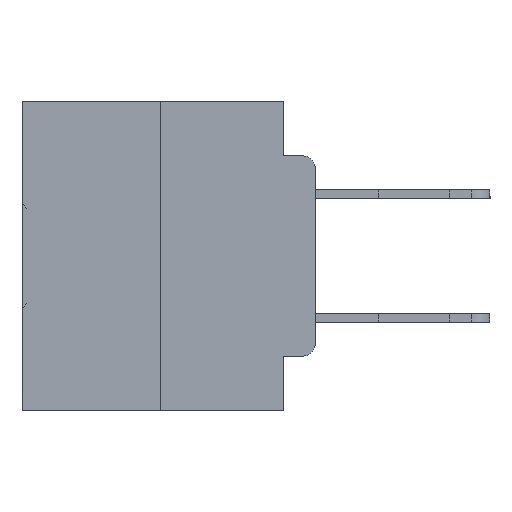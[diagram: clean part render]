
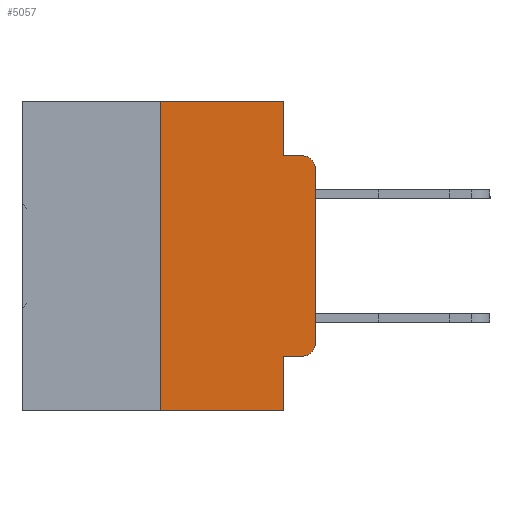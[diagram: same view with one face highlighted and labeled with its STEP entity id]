
A CAD part, left-side view. The second image highlights one B-rep face of the part: STEP entity #5057.
In plain terms, the highlighted planar face has unit normal (-1, 0, 0).
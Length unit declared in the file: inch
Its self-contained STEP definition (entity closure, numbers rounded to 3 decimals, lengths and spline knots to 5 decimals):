
#38 = VERTEX_POINT ( 'NONE', #27426 ) ;
#73 = EDGE_CURVE ( 'NONE', #22135, #20556, #468, .T. ) ;
#468 = CIRCLE ( 'NONE', #27942, 0.02 ) ;
#1991 = VERTEX_POINT ( 'NONE', #22120 ) ;
#2559 = DIRECTION ( 'NONE',  ( 0., 0., -1. ) ) ;
#2603 = CARTESIAN_POINT ( 'NONE',  ( 0., 0.02, -0.0885 ) ) ;
#2641 = VERTEX_POINT ( 'NONE', #11782 ) ;
#2790 = VECTOR ( 'NONE', #2559, 39.37008 ) ;
#3062 = ORIENTED_EDGE ( 'NONE', *, *, #28725, .F. ) ;
#3440 = CARTESIAN_POINT ( 'NONE',  ( 0., 0.25, 0. ) ) ;
#4510 = EDGE_CURVE ( 'NONE', #1991, #26244, #28996, .T. ) ;
#5057 = ADVANCED_FACE ( 'NONE', ( #19769 ), #16240, .F. ) ;
#5175 = ORIENTED_EDGE ( 'NONE', *, *, #10488, .F. ) ;
#5208 = CARTESIAN_POINT ( 'NONE',  ( 0., 0.02, -0.3915 ) ) ;
#5352 = CARTESIAN_POINT ( 'NONE',  ( 0., 0.051, 0. ) ) ;
#5661 = LINE ( 'NONE', #27698, #26513 ) ;
#6162 = ORIENTED_EDGE ( 'NONE', *, *, #22322, .T. ) ;
#6453 = EDGE_LOOP ( 'NONE', ( #10650, #28845, #28217, #3062, #5175, #31381, #14364, #29617, #17649, #6162 ) ) ;
#6769 = CARTESIAN_POINT ( 'NONE',  ( 0., 0.051, -0.4115 ) ) ;
#6932 = CIRCLE ( 'NONE', #30963, 0.02 ) ;
#7914 = DIRECTION ( 'NONE',  ( 0., 0., -1. ) ) ;
#8306 = VECTOR ( 'NONE', #17168, 39.37008 ) ;
#8898 = AXIS2_PLACEMENT_3D ( 'NONE', #13912, #11565, #14212 ) ;
#9503 = DIRECTION ( 'NONE',  ( 0., -1., 0. ) ) ;
#9935 = LINE ( 'NONE', #33737, #2790 ) ;
#10488 = EDGE_CURVE ( 'NONE', #26244, #26104, #29920, .T. ) ;
#10646 = DIRECTION ( 'NONE',  ( 0., -1., 0. ) ) ;
#10650 = ORIENTED_EDGE ( 'NONE', *, *, #28470, .T. ) ;
#11565 = DIRECTION ( 'NONE',  ( 1., 0., 0. ) ) ;
#11782 = CARTESIAN_POINT ( 'NONE',  ( 0., 0.02, -0.4115 ) ) ;
#12113 = VERTEX_POINT ( 'NONE', #20644 ) ;
#12252 = DIRECTION ( 'NONE',  ( 0., -1., 0. ) ) ;
#12771 = EDGE_CURVE ( 'NONE', #26099, #12113, #9935, .T. ) ;
#13738 = EDGE_CURVE ( 'NONE', #1991, #12113, #5661, .T. ) ;
#13912 = CARTESIAN_POINT ( 'NONE',  ( 0., 0.473, 0. ) ) ;
#14031 = CARTESIAN_POINT ( 'NONE',  ( 0., 0., -0.3915 ) ) ;
#14212 = DIRECTION ( 'NONE',  ( 0., 0., -1. ) ) ;
#14364 = ORIENTED_EDGE ( 'NONE', *, *, #13738, .T. ) ;
#14408 = DIRECTION ( 'NONE',  ( 0., -1., 0. ) ) ;
#14511 = LINE ( 'NONE', #6769, #20534 ) ;
#16130 = CARTESIAN_POINT ( 'NONE',  ( 0., 0.051, -0.4115 ) ) ;
#16240 = PLANE ( 'NONE',  #8898 ) ;
#17139 = CARTESIAN_POINT ( 'NONE',  ( 0., 0.25, 0. ) ) ;
#17168 = DIRECTION ( 'NONE',  ( 0., 0., 1. ) ) ;
#17247 = EDGE_CURVE ( 'NONE', #26099, #2641, #14511, .T. ) ;
#17649 = ORIENTED_EDGE ( 'NONE', *, *, #17247, .T. ) ;
#18200 = CARTESIAN_POINT ( 'NONE',  ( 0., 0., 0. ) ) ;
#19360 = VECTOR ( 'NONE', #10646, 39.37008 ) ;
#19769 = FACE_OUTER_BOUND ( 'NONE', #6453, .T. ) ;
#19830 = DIRECTION ( 'NONE',  ( 0., 0., -1. ) ) ;
#20383 = CARTESIAN_POINT ( 'NONE',  ( 0., 0.02, -0.1085 ) ) ;
#20534 = VECTOR ( 'NONE', #9503, 39.37008 ) ;
#20556 = VERTEX_POINT ( 'NONE', #2603 ) ;
#20644 = CARTESIAN_POINT ( 'NONE',  ( 0., 0.051, -0.5 ) ) ;
#20759 = DIRECTION ( 'NONE',  ( 0., 0., 1. ) ) ;
#22120 = CARTESIAN_POINT ( 'NONE',  ( 0., 0.25, -0.5 ) ) ;
#22135 = VERTEX_POINT ( 'NONE', #25374 ) ;
#22322 = EDGE_CURVE ( 'NONE', #2641, #29723, #6932, .T. ) ;
#23115 = VECTOR ( 'NONE', #14408, 39.37008 ) ;
#23562 = DIRECTION ( 'NONE',  ( -1., 0., 0. ) ) ;
#23589 = CARTESIAN_POINT ( 'NONE',  ( 0., 0.051, -0.0885 ) ) ;
#25374 = CARTESIAN_POINT ( 'NONE',  ( 0., 0., -0.1085 ) ) ;
#25826 = LINE ( 'NONE', #18200, #32574 ) ;
#26099 = VERTEX_POINT ( 'NONE', #16130 ) ;
#26104 = VERTEX_POINT ( 'NONE', #5352 ) ;
#26244 = VERTEX_POINT ( 'NONE', #3440 ) ;
#26513 = VECTOR ( 'NONE', #12252, 39.37008 ) ;
#26957 = LINE ( 'NONE', #23589, #19360 ) ;
#27425 = CARTESIAN_POINT ( 'NONE',  ( 0., 0.051, 0. ) ) ;
#27426 = CARTESIAN_POINT ( 'NONE',  ( 0., 0.051, -0.0885 ) ) ;
#27698 = CARTESIAN_POINT ( 'NONE',  ( 0., 0.473, -0.5 ) ) ;
#27942 = AXIS2_PLACEMENT_3D ( 'NONE', #20383, #29858, #31594 ) ;
#28217 = ORIENTED_EDGE ( 'NONE', *, *, #29554, .F. ) ;
#28470 = EDGE_CURVE ( 'NONE', #29723, #22135, #25826, .T. ) ;
#28725 = EDGE_CURVE ( 'NONE', #26104, #38, #31409, .T. ) ;
#28845 = ORIENTED_EDGE ( 'NONE', *, *, #73, .T. ) ;
#28996 = LINE ( 'NONE', #17139, #8306 ) ;
#29554 = EDGE_CURVE ( 'NONE', #38, #20556, #26957, .T. ) ;
#29617 = ORIENTED_EDGE ( 'NONE', *, *, #12771, .F. ) ;
#29723 = VERTEX_POINT ( 'NONE', #14031 ) ;
#29858 = DIRECTION ( 'NONE',  ( -1., 0., 0. ) ) ;
#29920 = LINE ( 'NONE', #32270, #23115 ) ;
#30603 = VECTOR ( 'NONE', #19830, 39.37008 ) ;
#30963 = AXIS2_PLACEMENT_3D ( 'NONE', #5208, #23562, #7914 ) ;
#31381 = ORIENTED_EDGE ( 'NONE', *, *, #4510, .F. ) ;
#31409 = LINE ( 'NONE', #27425, #30603 ) ;
#31594 = DIRECTION ( 'NONE',  ( 0., 0., -1. ) ) ;
#32270 = CARTESIAN_POINT ( 'NONE',  ( 0., 0.473, 0. ) ) ;
#32574 = VECTOR ( 'NONE', #20759, 39.37008 ) ;
#33737 = CARTESIAN_POINT ( 'NONE',  ( 0., 0.051, 0. ) ) ;
